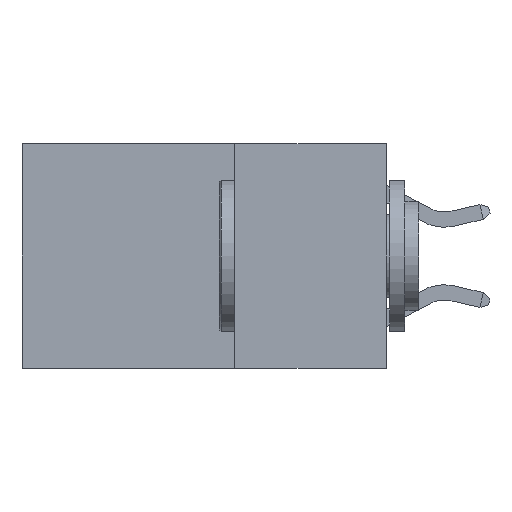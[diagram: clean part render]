
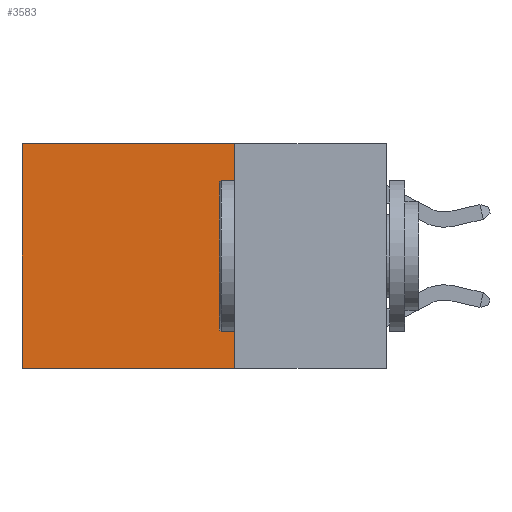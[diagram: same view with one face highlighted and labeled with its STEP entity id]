
A CAD part, left-side view. The second image highlights one B-rep face of the part: STEP entity #3583.
In plain terms, the highlighted planar face has unit normal (-1, 0, 0).
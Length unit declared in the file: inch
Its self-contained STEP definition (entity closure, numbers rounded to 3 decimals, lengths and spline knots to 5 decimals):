
#291 = DIRECTION ( 'NONE',  ( 0., 1., 0. ) ) ;
#905 = EDGE_LOOP ( 'NONE', ( #10435, #10042, #7254, #5195 ) ) ;
#1084 = EDGE_CURVE ( 'NONE', #6581, #3400, #2664, .T. ) ;
#2664 = LINE ( 'NONE', #9311, #3287 ) ;
#2711 = VECTOR ( 'NONE', #8365, 39.37008 ) ;
#2987 = PLANE ( 'NONE',  #8099 ) ;
#3031 = DIRECTION ( 'NONE',  ( 0., 0., -1. ) ) ;
#3287 = VECTOR ( 'NONE', #291, 39.37008 ) ;
#3400 = VERTEX_POINT ( 'NONE', #5396 ) ;
#3583 = ADVANCED_FACE ( 'NONE', ( #7342 ), #2987, .F. ) ;
#3881 = VERTEX_POINT ( 'NONE', #9578 ) ;
#4423 = LINE ( 'NONE', #11670, #5041 ) ;
#4683 = EDGE_CURVE ( 'NONE', #3881, #5738, #8091, .T. ) ;
#5041 = VECTOR ( 'NONE', #5769, 39.37008 ) ;
#5195 = ORIENTED_EDGE ( 'NONE', *, *, #4683, .T. ) ;
#5396 = CARTESIAN_POINT ( 'NONE',  ( 0.2625, 0.6, -0.37 ) ) ;
#5689 = VECTOR ( 'NONE', #9629, 39.37008 ) ;
#5738 = VERTEX_POINT ( 'NONE', #8644 ) ;
#5761 = CARTESIAN_POINT ( 'NONE',  ( 0.2625, 0.6, 0. ) ) ;
#5769 = DIRECTION ( 'NONE',  ( 0., 0., -1. ) ) ;
#6581 = VERTEX_POINT ( 'NONE', #10717 ) ;
#6667 = EDGE_CURVE ( 'NONE', #3881, #6581, #4423, .T. ) ;
#7254 = ORIENTED_EDGE ( 'NONE', *, *, #6667, .F. ) ;
#7342 = FACE_OUTER_BOUND ( 'NONE', #905, .T. ) ;
#8091 = LINE ( 'NONE', #11315, #2711 ) ;
#8099 = AXIS2_PLACEMENT_3D ( 'NONE', #10784, #9695, #3031 ) ;
#8365 = DIRECTION ( 'NONE',  ( 0., 1., 0. ) ) ;
#8644 = CARTESIAN_POINT ( 'NONE',  ( 0.2625, 0.6, 0. ) ) ;
#9221 = EDGE_CURVE ( 'NONE', #5738, #3400, #12173, .T. ) ;
#9311 = CARTESIAN_POINT ( 'NONE',  ( 0.2625, 0.25, -0.37 ) ) ;
#9578 = CARTESIAN_POINT ( 'NONE',  ( 0.2625, 0.25, 0. ) ) ;
#9629 = DIRECTION ( 'NONE',  ( 0., 0., -1. ) ) ;
#9695 = DIRECTION ( 'NONE',  ( 1., 0., 0. ) ) ;
#10042 = ORIENTED_EDGE ( 'NONE', *, *, #1084, .F. ) ;
#10435 = ORIENTED_EDGE ( 'NONE', *, *, #9221, .T. ) ;
#10717 = CARTESIAN_POINT ( 'NONE',  ( 0.2625, 0.25, -0.37 ) ) ;
#10784 = CARTESIAN_POINT ( 'NONE',  ( 0.2625, 0.25, 0. ) ) ;
#11315 = CARTESIAN_POINT ( 'NONE',  ( 0.2625, 0.25, 0. ) ) ;
#11670 = CARTESIAN_POINT ( 'NONE',  ( 0.2625, 0.25, 0. ) ) ;
#12173 = LINE ( 'NONE', #5761, #5689 ) ;
